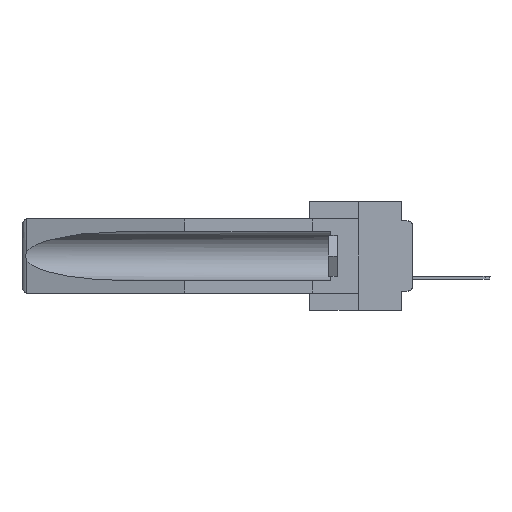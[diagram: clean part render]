
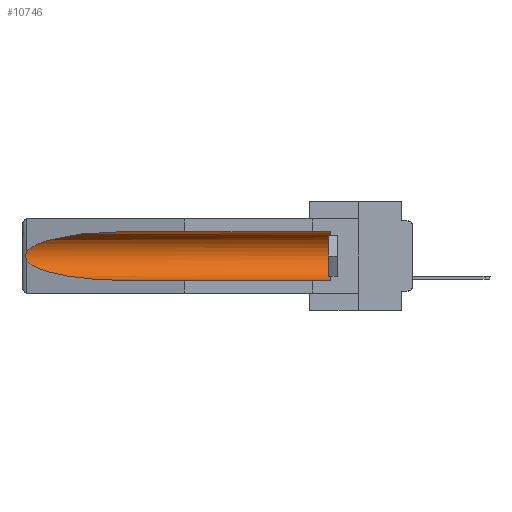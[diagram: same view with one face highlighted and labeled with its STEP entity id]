
A CAD part, left-side view. The second image highlights one B-rep face of the part: STEP entity #10746.
In plain terms, the highlighted cylindrical face has radius 2.857 mm (diameter 5.715 mm), a partial arc.
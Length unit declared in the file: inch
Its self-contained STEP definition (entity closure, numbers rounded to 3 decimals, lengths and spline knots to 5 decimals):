
#47 = EDGE_CURVE ( 'NONE', #17954, #10747, #15627, .T. ) ;
#156 = DIRECTION ( 'NONE',  ( 0., 1., 0. ) ) ;
#255 = VERTEX_POINT ( 'NONE', #19312 ) ;
#1379 = VERTEX_POINT ( 'NONE', #29277 ) ;
#1465 = CARTESIAN_POINT ( 'NONE',  ( 0.26537, 1.52718, -0.19328 ) ) ;
#1543 = CARTESIAN_POINT ( 'NONE',  ( 0.155, 1.07973, -0.059 ) ) ;
#2412 = DIRECTION ( 'NONE',  ( 0., 1., 0. ) ) ;
#3454 = CARTESIAN_POINT ( 'NONE',  ( 0.26597, 1.5296, -0.19026 ) ) ;
#3867 = CARTESIAN_POINT ( 'NONE',  ( 0.26597, 1.52961, -0.15275 ) ) ;
#4368 = CYLINDRICAL_SURFACE ( 'NONE', #20152, 0.1125 ) ;
#4675 = CARTESIAN_POINT ( 'NONE',  ( 0.21114, 1.30732, -0.284 ) ) ;
#4969 =( BOUNDED_CURVE ( )  B_SPLINE_CURVE ( 3, ( #23269, #25677, #25384, #23083 ),
 .UNSPECIFIED., .F., .T. ) 
 B_SPLINE_CURVE_WITH_KNOTS ( ( 4, 4 ),
 ( 4.71239, 6.08839 ),
 .UNSPECIFIED. ) 
 CURVE ( )  GEOMETRIC_REPRESENTATION_ITEM ( )  RATIONAL_B_SPLINE_CURVE ( ( 1., 0.848, 0.848, 1. ) ) 
 REPRESENTATION_ITEM ( '' )  );
#5139 = ORIENTED_EDGE ( 'NONE', *, *, #18709, .T. ) ;
#5577 = EDGE_CURVE ( 'NONE', #1379, #10747, #16244, .T. ) ;
#5935 = CARTESIAN_POINT ( 'NONE',  ( 0.2673, 1.5327, -0.16383 ) ) ;
#5960 = VERTEX_POINT ( 'NONE', #1543 ) ;
#6729 = EDGE_CURVE ( 'NONE', #13406, #5960, #7224, .T. ) ;
#7224 = LINE ( 'NONE', #24562, #19373 ) ;
#8659 = DIRECTION ( 'NONE',  ( 0., 1., 0. ) ) ;
#9364 = CARTESIAN_POINT ( 'NONE',  ( 0.155, 1.07973, -0.284 ) ) ;
#9978 = ORIENTED_EDGE ( 'NONE', *, *, #6729, .T. ) ;
#10746 = ADVANCED_FACE ( 'NONE', ( #13669 ), #4368, .F. ) ;
#10747 = VERTEX_POINT ( 'NONE', #9364 ) ;
#11753 = B_SPLINE_CURVE_WITH_KNOTS ( 'NONE', 3,
 ( #28535, #3867, #28634, #5935, #21713, #15172, #14980, #26428, #3454, #1465 ),
 .UNSPECIFIED., .F., .F.,
 ( 4, 2, 2, 2, 4 ),
 ( 0., 0.00029, 0.00058, 0.00087, 0.00117 ),
 .UNSPECIFIED. ) ;
#13095 = ORIENTED_EDGE ( 'NONE', *, *, #17302, .T. ) ;
#13288 = CARTESIAN_POINT ( 'NONE',  ( 0.25451, 1.48313, -0.24835 ) ) ;
#13406 = VERTEX_POINT ( 'NONE', #15879 ) ;
#13484 = EDGE_LOOP ( 'NONE', ( #13095, #25247, #13960, #20344, #5139, #9978 ) ) ;
#13669 = FACE_OUTER_BOUND ( 'NONE', #13484, .T. ) ;
#13875 = CARTESIAN_POINT ( 'NONE',  ( 0.155, -0.30754, -0.1715 ) ) ;
#13960 = ORIENTED_EDGE ( 'NONE', *, *, #47, .T. ) ;
#14835 = VECTOR ( 'NONE', #2412, 39.37008 ) ;
#14980 = CARTESIAN_POINT ( 'NONE',  ( 0.2673, 1.53269, -0.17917 ) ) ;
#15172 = CARTESIAN_POINT ( 'NONE',  ( 0.2675, 1.53308, -0.17534 ) ) ;
#15627 =( BOUNDED_CURVE ( )  B_SPLINE_CURVE ( 3, ( #19931, #13288, #4675, #27465 ),
 .UNSPECIFIED., .F., .F. ) 
 B_SPLINE_CURVE_WITH_KNOTS ( ( 4, 4 ),
 ( 0.1948, 1.5708 ),
 .UNSPECIFIED. ) 
 CURVE ( )  GEOMETRIC_REPRESENTATION_ITEM ( )  RATIONAL_B_SPLINE_CURVE ( ( 1., 0.848, 0.848, 1. ) ) 
 REPRESENTATION_ITEM ( '' )  );
#15879 = CARTESIAN_POINT ( 'NONE',  ( 0.155, 0.126, -0.059 ) ) ;
#16244 = LINE ( 'NONE', #21374, #14835 ) ;
#16500 = DIRECTION ( 'NONE',  ( 0., -1., 0. ) ) ;
#17302 = EDGE_CURVE ( 'NONE', #5960, #255, #4969, .T. ) ;
#17954 = VERTEX_POINT ( 'NONE', #21133 ) ;
#18709 = EDGE_CURVE ( 'NONE', #1379, #13406, #20016, .T. ) ;
#19312 = CARTESIAN_POINT ( 'NONE',  ( 0.26537, 1.52718, -0.14972 ) ) ;
#19373 = VECTOR ( 'NONE', #8659, 39.37008 ) ;
#19931 = CARTESIAN_POINT ( 'NONE',  ( 0.26537, 1.52718, -0.19328 ) ) ;
#20016 = CIRCLE ( 'NONE', #29599, 0.1125 ) ;
#20152 = AXIS2_PLACEMENT_3D ( 'NONE', #13875, #156, #23023 ) ;
#20344 = ORIENTED_EDGE ( 'NONE', *, *, #5577, .F. ) ;
#21133 = CARTESIAN_POINT ( 'NONE',  ( 0.26537, 1.52718, -0.19328 ) ) ;
#21367 = DIRECTION ( 'NONE',  ( 0., 0., 1. ) ) ;
#21374 = CARTESIAN_POINT ( 'NONE',  ( 0.155, -0.30754, -0.284 ) ) ;
#21713 = CARTESIAN_POINT ( 'NONE',  ( 0.2675, 1.53308, -0.16763 ) ) ;
#23023 = DIRECTION ( 'NONE',  ( 0., 0., 1. ) ) ;
#23083 = CARTESIAN_POINT ( 'NONE',  ( 0.26537, 1.52718, -0.14972 ) ) ;
#23269 = CARTESIAN_POINT ( 'NONE',  ( 0.155, 1.07973, -0.059 ) ) ;
#24562 = CARTESIAN_POINT ( 'NONE',  ( 0.155, -0.30754, -0.059 ) ) ;
#25247 = ORIENTED_EDGE ( 'NONE', *, *, #26452, .T. ) ;
#25384 = CARTESIAN_POINT ( 'NONE',  ( 0.25451, 1.48313, -0.09465 ) ) ;
#25677 = CARTESIAN_POINT ( 'NONE',  ( 0.21114, 1.30732, -0.059 ) ) ;
#26428 = CARTESIAN_POINT ( 'NONE',  ( 0.26655, 1.53094, -0.18657 ) ) ;
#26452 = EDGE_CURVE ( 'NONE', #255, #17954, #11753, .T. ) ;
#27465 = CARTESIAN_POINT ( 'NONE',  ( 0.155, 1.07973, -0.284 ) ) ;
#27910 = CARTESIAN_POINT ( 'NONE',  ( 0.155, 0.126, -0.1715 ) ) ;
#28535 = CARTESIAN_POINT ( 'NONE',  ( 0.26537, 1.52718, -0.14972 ) ) ;
#28634 = CARTESIAN_POINT ( 'NONE',  ( 0.26654, 1.53092, -0.15636 ) ) ;
#29277 = CARTESIAN_POINT ( 'NONE',  ( 0.155, 0.126, -0.284 ) ) ;
#29599 = AXIS2_PLACEMENT_3D ( 'NONE', #27910, #16500, #21367 ) ;
